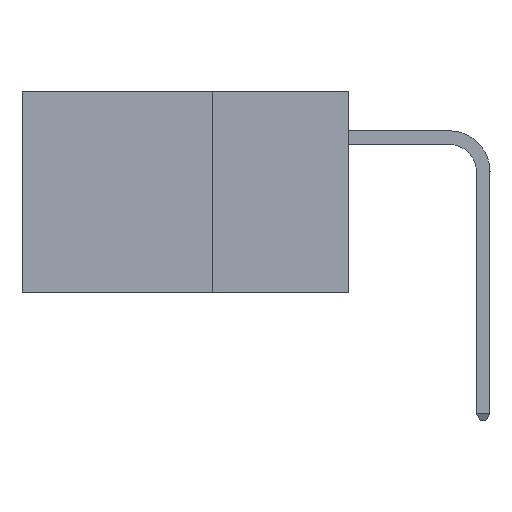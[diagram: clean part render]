
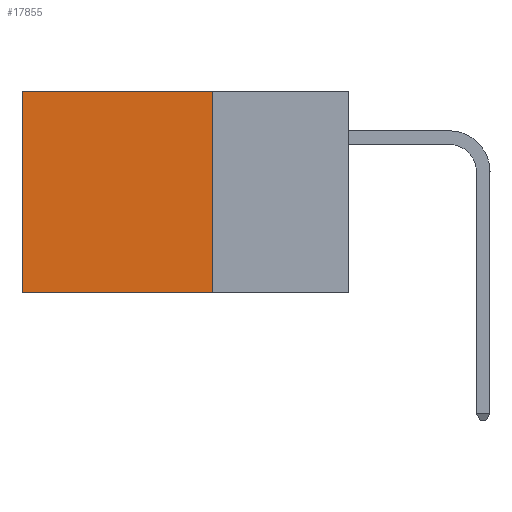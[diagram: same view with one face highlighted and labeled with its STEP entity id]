
A CAD part, left-side view. The second image highlights one B-rep face of the part: STEP entity #17855.
In plain terms, the highlighted planar face has unit normal (-1, 0, 0).
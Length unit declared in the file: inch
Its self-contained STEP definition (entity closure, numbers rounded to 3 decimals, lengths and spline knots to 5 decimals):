
#1233 = VERTEX_POINT ( 'NONE', #14646 ) ;
#1483 = ORIENTED_EDGE ( 'NONE', *, *, #4428, .F. ) ;
#3699 = ORIENTED_EDGE ( 'NONE', *, *, #39265, .T. ) ;
#4428 = EDGE_CURVE ( 'NONE', #32551, #30578, #10242, .T. ) ;
#4747 = VERTEX_POINT ( 'NONE', #20530 ) ;
#7241 = ORIENTED_EDGE ( 'NONE', *, *, #11872, .F. ) ;
#7731 = DIRECTION ( 'NONE',  ( 0., 1., 0. ) ) ;
#8855 = CARTESIAN_POINT ( 'NONE',  ( 0.2875, 0.6, -0.37 ) ) ;
#10242 = LINE ( 'NONE', #35682, #34660 ) ;
#10726 = VECTOR ( 'NONE', #32812, 39.37008 ) ;
#11522 = DIRECTION ( 'NONE',  ( 0., 0., -1. ) ) ;
#11872 = EDGE_CURVE ( 'NONE', #1233, #32551, #16455, .T. ) ;
#14646 = CARTESIAN_POINT ( 'NONE',  ( 0.2875, 0.25, 0. ) ) ;
#14777 = LINE ( 'NONE', #34013, #37257 ) ;
#16455 = LINE ( 'NONE', #32189, #10726 ) ;
#17855 = ADVANCED_FACE ( 'NONE', ( #24551 ), #20540, .F. ) ;
#18502 = DIRECTION ( 'NONE',  ( 1., 0., 0. ) ) ;
#20356 = EDGE_LOOP ( 'NONE', ( #3699, #1483, #7241, #22749 ) ) ;
#20530 = CARTESIAN_POINT ( 'NONE',  ( 0.2875, 0.6, 0. ) ) ;
#20540 = PLANE ( 'NONE',  #35990 ) ;
#21208 = CARTESIAN_POINT ( 'NONE',  ( 0.2875, 0.25, 0. ) ) ;
#22749 = ORIENTED_EDGE ( 'NONE', *, *, #36138, .T. ) ;
#23932 = CARTESIAN_POINT ( 'NONE',  ( 0.2875, 0.6, 0. ) ) ;
#24551 = FACE_OUTER_BOUND ( 'NONE', #20356, .T. ) ;
#24882 = DIRECTION ( 'NONE',  ( 0., 1., 0. ) ) ;
#26750 = VECTOR ( 'NONE', #11522, 39.37008 ) ;
#27047 = CARTESIAN_POINT ( 'NONE',  ( 0.2875, 0.25, -0.37 ) ) ;
#27409 = DIRECTION ( 'NONE',  ( 0., 0., -1. ) ) ;
#30578 = VERTEX_POINT ( 'NONE', #8855 ) ;
#32189 = CARTESIAN_POINT ( 'NONE',  ( 0.2875, 0.25, 0. ) ) ;
#32506 = LINE ( 'NONE', #23932, #26750 ) ;
#32551 = VERTEX_POINT ( 'NONE', #27047 ) ;
#32812 = DIRECTION ( 'NONE',  ( 0., 0., -1. ) ) ;
#34013 = CARTESIAN_POINT ( 'NONE',  ( 0.2875, 0.25, 0. ) ) ;
#34660 = VECTOR ( 'NONE', #7731, 39.37008 ) ;
#35682 = CARTESIAN_POINT ( 'NONE',  ( 0.2875, 0.25, -0.37 ) ) ;
#35990 = AXIS2_PLACEMENT_3D ( 'NONE', #21208, #18502, #27409 ) ;
#36138 = EDGE_CURVE ( 'NONE', #1233, #4747, #14777, .T. ) ;
#37257 = VECTOR ( 'NONE', #24882, 39.37008 ) ;
#39265 = EDGE_CURVE ( 'NONE', #4747, #30578, #32506, .T. ) ;
